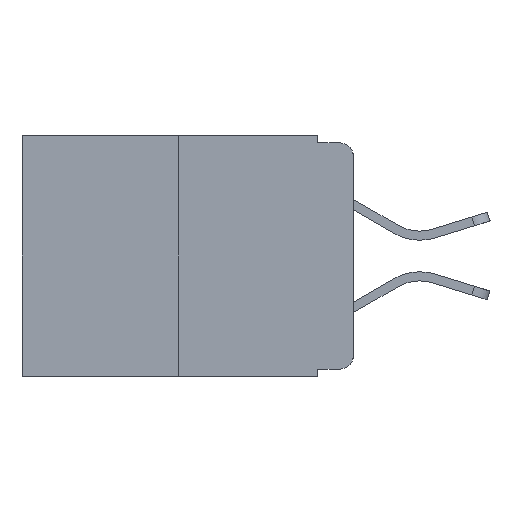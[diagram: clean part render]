
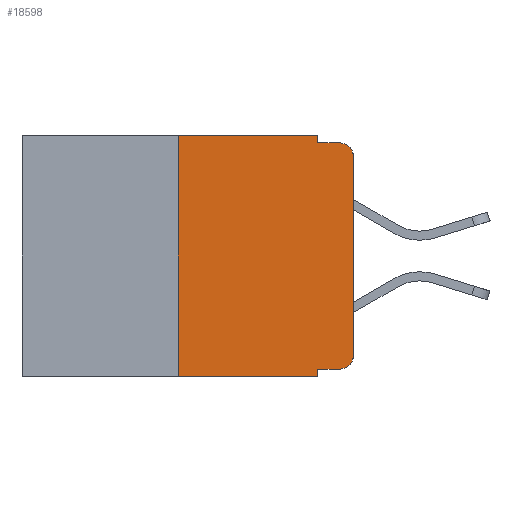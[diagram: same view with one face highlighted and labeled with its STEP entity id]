
A CAD part, left-side view. The second image highlights one B-rep face of the part: STEP entity #18598.
In plain terms, the highlighted planar face has unit normal (-1, 0, 0).
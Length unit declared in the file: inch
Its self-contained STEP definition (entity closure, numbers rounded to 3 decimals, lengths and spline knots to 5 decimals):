
#765 = ORIENTED_EDGE ( 'NONE', *, *, #11616, .F. ) ;
#906 = CARTESIAN_POINT ( 'NONE',  ( 0., 0.02, -0.01 ) ) ;
#1227 = VECTOR ( 'NONE', #14620, 39.37008 ) ;
#1825 = CARTESIAN_POINT ( 'NONE',  ( 0., 0.473, -0.343 ) ) ;
#2141 = EDGE_CURVE ( 'NONE', #14466, #23223, #19071, .T. ) ;
#2182 = ORIENTED_EDGE ( 'NONE', *, *, #3430, .T. ) ;
#2497 = ORIENTED_EDGE ( 'NONE', *, *, #9195, .F. ) ;
#2512 = CARTESIAN_POINT ( 'NONE',  ( 0., 0., -0.313 ) ) ;
#2769 = ORIENTED_EDGE ( 'NONE', *, *, #20821, .T. ) ;
#2783 = CARTESIAN_POINT ( 'NONE',  ( 0., 0.051, -0.01 ) ) ;
#2818 = EDGE_CURVE ( 'NONE', #14313, #3398, #5447, .T. ) ;
#3398 = VERTEX_POINT ( 'NONE', #16275 ) ;
#3430 = EDGE_CURVE ( 'NONE', #15886, #20397, #12309, .T. ) ;
#3681 = ORIENTED_EDGE ( 'NONE', *, *, #12813, .F. ) ;
#4095 = FACE_OUTER_BOUND ( 'NONE', #5236, .T. ) ;
#4841 = VECTOR ( 'NONE', #19205, 39.37008 ) ;
#5120 = AXIS2_PLACEMENT_3D ( 'NONE', #12645, #9101, #21368 ) ;
#5236 = EDGE_LOOP ( 'NONE', ( #2182, #2769, #22954, #2497, #17727, #765, #21589, #3681, #18560, #19104 ) ) ;
#5447 = LINE ( 'NONE', #17944, #14520 ) ;
#5656 = CARTESIAN_POINT ( 'NONE',  ( 0., 0.051, -0.343 ) ) ;
#7072 = CARTESIAN_POINT ( 'NONE',  ( 0., 0.25, 0. ) ) ;
#7772 = VERTEX_POINT ( 'NONE', #5656 ) ;
#7804 = EDGE_CURVE ( 'NONE', #17135, #14306, #8882, .T. ) ;
#8781 = DIRECTION ( 'NONE',  ( 0., -1., 0. ) ) ;
#8882 = LINE ( 'NONE', #21735, #21783 ) ;
#8933 = DIRECTION ( 'NONE',  ( 0., 0., 1. ) ) ;
#8934 = CARTESIAN_POINT ( 'NONE',  ( 0., 0.02, -0.333 ) ) ;
#9062 = EDGE_CURVE ( 'NONE', #15450, #7772, #20340, .T. ) ;
#9101 = DIRECTION ( 'NONE',  ( 1., 0., 0. ) ) ;
#9195 = EDGE_CURVE ( 'NONE', #3398, #17135, #13029, .T. ) ;
#9368 = AXIS2_PLACEMENT_3D ( 'NONE', #10253, #22482, #12038 ) ;
#9645 = CARTESIAN_POINT ( 'NONE',  ( 0., 0.051, 0. ) ) ;
#9763 = DIRECTION ( 'NONE',  ( -1., 0., 0. ) ) ;
#10253 = CARTESIAN_POINT ( 'NONE',  ( 0., 0.02, -0.03 ) ) ;
#10660 = CARTESIAN_POINT ( 'NONE',  ( 0., 0.051, -0.333 ) ) ;
#11616 = EDGE_CURVE ( 'NONE', #15450, #14313, #21069, .T. ) ;
#11843 = CIRCLE ( 'NONE', #9368, 0.02 ) ;
#12038 = DIRECTION ( 'NONE',  ( 0., 0., -1. ) ) ;
#12309 = LINE ( 'NONE', #14568, #17450 ) ;
#12645 = CARTESIAN_POINT ( 'NONE',  ( 0., 0.473, 0. ) ) ;
#12813 = EDGE_CURVE ( 'NONE', #14466, #7772, #19909, .T. ) ;
#13029 = LINE ( 'NONE', #9645, #15749 ) ;
#13073 = DIRECTION ( 'NONE',  ( 0., -1., 0. ) ) ;
#14306 = VERTEX_POINT ( 'NONE', #906 ) ;
#14313 = VERTEX_POINT ( 'NONE', #15490 ) ;
#14466 = VERTEX_POINT ( 'NONE', #10660 ) ;
#14520 = VECTOR ( 'NONE', #8781, 39.37008 ) ;
#14561 = DIRECTION ( 'NONE',  ( 0., 0., 1. ) ) ;
#14568 = CARTESIAN_POINT ( 'NONE',  ( 0., 0., 0. ) ) ;
#14620 = DIRECTION ( 'NONE',  ( 0., -1., 0. ) ) ;
#15334 = VECTOR ( 'NONE', #16149, 39.37008 ) ;
#15450 = VERTEX_POINT ( 'NONE', #18802 ) ;
#15490 = CARTESIAN_POINT ( 'NONE',  ( 0., 0.25, 0. ) ) ;
#15749 = VECTOR ( 'NONE', #20104, 39.37008 ) ;
#15886 = VERTEX_POINT ( 'NONE', #2512 ) ;
#15891 = VECTOR ( 'NONE', #8933, 39.37008 ) ;
#16027 = CARTESIAN_POINT ( 'NONE',  ( 0., 0., -0.03 ) ) ;
#16149 = DIRECTION ( 'NONE',  ( 0., 0., -1. ) ) ;
#16275 = CARTESIAN_POINT ( 'NONE',  ( 0., 0.051, 0. ) ) ;
#17135 = VERTEX_POINT ( 'NONE', #2783 ) ;
#17450 = VECTOR ( 'NONE', #14561, 39.37008 ) ;
#17727 = ORIENTED_EDGE ( 'NONE', *, *, #2818, .F. ) ;
#17944 = CARTESIAN_POINT ( 'NONE',  ( 0., 0.473, 0. ) ) ;
#18395 = CARTESIAN_POINT ( 'NONE',  ( 0., 0.051, -0.333 ) ) ;
#18560 = ORIENTED_EDGE ( 'NONE', *, *, #2141, .T. ) ;
#18598 = ADVANCED_FACE ( 'NONE', ( #4095 ), #19577, .F. ) ;
#18802 = CARTESIAN_POINT ( 'NONE',  ( 0., 0.25, -0.343 ) ) ;
#18851 = CIRCLE ( 'NONE', #19167, 0.02 ) ;
#19071 = LINE ( 'NONE', #18395, #4841 ) ;
#19104 = ORIENTED_EDGE ( 'NONE', *, *, #20651, .T. ) ;
#19167 = AXIS2_PLACEMENT_3D ( 'NONE', #20227, #9763, #22018 ) ;
#19205 = DIRECTION ( 'NONE',  ( 0., -1., 0. ) ) ;
#19577 = PLANE ( 'NONE',  #5120 ) ;
#19909 = LINE ( 'NONE', #21316, #15334 ) ;
#20104 = DIRECTION ( 'NONE',  ( 0., 0., -1. ) ) ;
#20227 = CARTESIAN_POINT ( 'NONE',  ( 0., 0.02, -0.313 ) ) ;
#20340 = LINE ( 'NONE', #1825, #1227 ) ;
#20397 = VERTEX_POINT ( 'NONE', #16027 ) ;
#20651 = EDGE_CURVE ( 'NONE', #23223, #15886, #18851, .T. ) ;
#20821 = EDGE_CURVE ( 'NONE', #20397, #14306, #11843, .T. ) ;
#21069 = LINE ( 'NONE', #7072, #15891 ) ;
#21316 = CARTESIAN_POINT ( 'NONE',  ( 0., 0.051, 0. ) ) ;
#21368 = DIRECTION ( 'NONE',  ( 0., 0., -1. ) ) ;
#21589 = ORIENTED_EDGE ( 'NONE', *, *, #9062, .T. ) ;
#21735 = CARTESIAN_POINT ( 'NONE',  ( 0., 0.051, -0.01 ) ) ;
#21783 = VECTOR ( 'NONE', #13073, 39.37008 ) ;
#22018 = DIRECTION ( 'NONE',  ( 0., 0., -1. ) ) ;
#22482 = DIRECTION ( 'NONE',  ( -1., 0., 0. ) ) ;
#22954 = ORIENTED_EDGE ( 'NONE', *, *, #7804, .F. ) ;
#23223 = VERTEX_POINT ( 'NONE', #8934 ) ;
